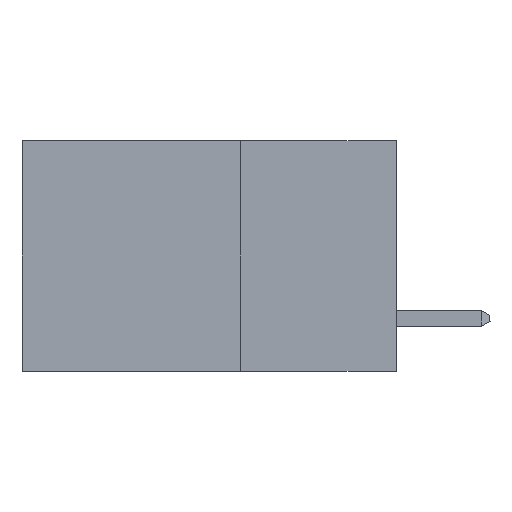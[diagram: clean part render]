
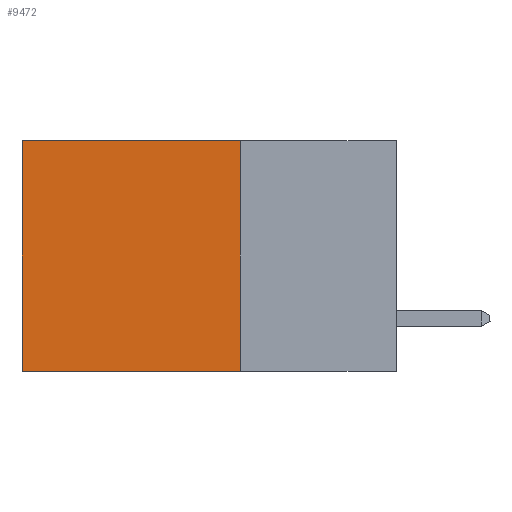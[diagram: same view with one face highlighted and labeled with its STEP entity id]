
A CAD part, left-side view. The second image highlights one B-rep face of the part: STEP entity #9472.
In plain terms, the highlighted planar face has unit normal (-1, 0, 0).
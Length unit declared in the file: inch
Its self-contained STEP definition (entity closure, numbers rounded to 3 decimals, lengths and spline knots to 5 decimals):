
#163 = ORIENTED_EDGE ( 'NONE', *, *, #11644, .T. ) ;
#317 = VERTEX_POINT ( 'NONE', #4002 ) ;
#460 = VECTOR ( 'NONE', #6882, 39.37008 ) ;
#578 = DIRECTION ( 'NONE',  ( 0., 1., 0. ) ) ;
#950 = AXIS2_PLACEMENT_3D ( 'NONE', #5499, #8330, #2590 ) ;
#1103 = CARTESIAN_POINT ( 'NONE',  ( 0.298, 0.6, 0. ) ) ;
#1136 = VERTEX_POINT ( 'NONE', #4183 ) ;
#1646 = VECTOR ( 'NONE', #10411, 39.37008 ) ;
#2008 = CARTESIAN_POINT ( 'NONE',  ( 0.298, 0.6, -0.37 ) ) ;
#2590 = DIRECTION ( 'NONE',  ( 0., 0., -1. ) ) ;
#3880 = CARTESIAN_POINT ( 'NONE',  ( 0.298, 0.25, 0. ) ) ;
#4002 = CARTESIAN_POINT ( 'NONE',  ( 0.298, 0.6, 0. ) ) ;
#4110 = DIRECTION ( 'NONE',  ( 0., 0., -1. ) ) ;
#4183 = CARTESIAN_POINT ( 'NONE',  ( 0.298, 0.25, -0.37 ) ) ;
#4205 = LINE ( 'NONE', #9467, #1646 ) ;
#4375 = ORIENTED_EDGE ( 'NONE', *, *, #10256, .T. ) ;
#5224 = LINE ( 'NONE', #1103, #460 ) ;
#5499 = CARTESIAN_POINT ( 'NONE',  ( 0.298, 0.25, 0. ) ) ;
#5984 = CARTESIAN_POINT ( 'NONE',  ( 0.298, 0.25, 0. ) ) ;
#5990 = FACE_OUTER_BOUND ( 'NONE', #9611, .T. ) ;
#6452 = PLANE ( 'NONE',  #950 ) ;
#6623 = VERTEX_POINT ( 'NONE', #2008 ) ;
#6846 = LINE ( 'NONE', #11835, #8999 ) ;
#6882 = DIRECTION ( 'NONE',  ( 0., 0., -1. ) ) ;
#7257 = EDGE_CURVE ( 'NONE', #9133, #1136, #9813, .T. ) ;
#8330 = DIRECTION ( 'NONE',  ( 1., 0., 0. ) ) ;
#8999 = VECTOR ( 'NONE', #578, 39.37008 ) ;
#9069 = ORIENTED_EDGE ( 'NONE', *, *, #12159, .F. ) ;
#9133 = VERTEX_POINT ( 'NONE', #3880 ) ;
#9467 = CARTESIAN_POINT ( 'NONE',  ( 0.298, 0.25, 0. ) ) ;
#9472 = ADVANCED_FACE ( 'NONE', ( #5990 ), #6452, .F. ) ;
#9508 = VECTOR ( 'NONE', #4110, 39.37008 ) ;
#9611 = EDGE_LOOP ( 'NONE', ( #163, #9069, #10429, #4375 ) ) ;
#9813 = LINE ( 'NONE', #5984, #9508 ) ;
#10256 = EDGE_CURVE ( 'NONE', #9133, #317, #4205, .T. ) ;
#10411 = DIRECTION ( 'NONE',  ( 0., 1., 0. ) ) ;
#10429 = ORIENTED_EDGE ( 'NONE', *, *, #7257, .F. ) ;
#11644 = EDGE_CURVE ( 'NONE', #317, #6623, #5224, .T. ) ;
#11835 = CARTESIAN_POINT ( 'NONE',  ( 0.298, 0.25, -0.37 ) ) ;
#12159 = EDGE_CURVE ( 'NONE', #1136, #6623, #6846, .T. ) ;
